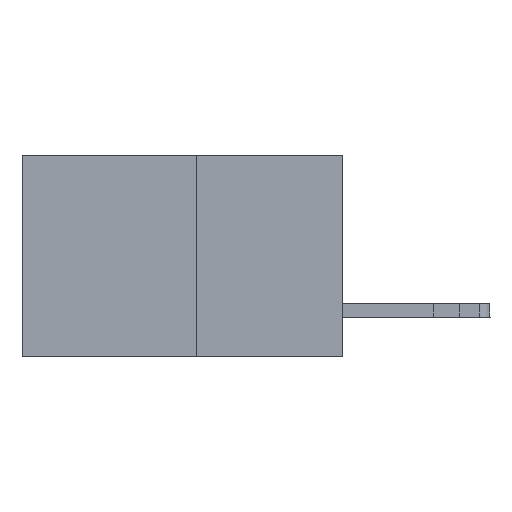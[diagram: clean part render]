
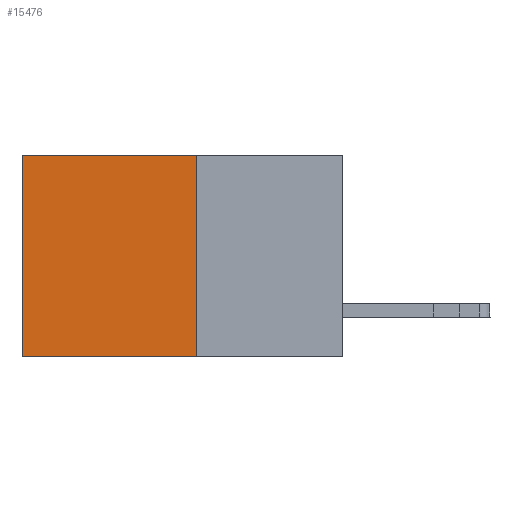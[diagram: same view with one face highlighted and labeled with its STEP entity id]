
A CAD part, left-side view. The second image highlights one B-rep face of the part: STEP entity #15476.
In plain terms, the highlighted planar face has unit normal (-1, 0, 0).
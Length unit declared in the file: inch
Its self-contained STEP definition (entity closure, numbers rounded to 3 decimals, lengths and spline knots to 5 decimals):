
#254 = EDGE_CURVE ( 'NONE', #26780, #20429, #19326, .T. ) ;
#1365 = VERTEX_POINT ( 'NONE', #3484 ) ;
#2814 = LINE ( 'NONE', #14311, #10953 ) ;
#2864 = EDGE_LOOP ( 'NONE', ( #21730, #12178, #21146, #21820 ) ) ;
#3484 = CARTESIAN_POINT ( 'NONE',  ( 0.277, 0.59, 0. ) ) ;
#6136 = VERTEX_POINT ( 'NONE', #21966 ) ;
#7174 = CARTESIAN_POINT ( 'NONE',  ( 0.277, 0.27, -0.37 ) ) ;
#8722 = CARTESIAN_POINT ( 'NONE',  ( 0.277, 0.27, -0.37 ) ) ;
#8841 = EDGE_CURVE ( 'NONE', #1365, #6136, #2814, .T. ) ;
#8931 = EDGE_CURVE ( 'NONE', #20429, #6136, #26790, .T. ) ;
#9670 = DIRECTION ( 'NONE',  ( 0., 1., 0. ) ) ;
#9918 = DIRECTION ( 'NONE',  ( 0., 1., 0. ) ) ;
#10953 = VECTOR ( 'NONE', #31587, 39.37008 ) ;
#11965 = EDGE_CURVE ( 'NONE', #26780, #1365, #26140, .T. ) ;
#12178 = ORIENTED_EDGE ( 'NONE', *, *, #8931, .F. ) ;
#12986 = VECTOR ( 'NONE', #9918, 39.37008 ) ;
#14311 = CARTESIAN_POINT ( 'NONE',  ( 0.277, 0.59, -0.37 ) ) ;
#14788 = CARTESIAN_POINT ( 'NONE',  ( 0.277, 0.27, 0. ) ) ;
#15362 = AXIS2_PLACEMENT_3D ( 'NONE', #22128, #19560, #27088 ) ;
#15476 = ADVANCED_FACE ( 'NONE', ( #15917 ), #24604, .F. ) ;
#15917 = FACE_OUTER_BOUND ( 'NONE', #2864, .T. ) ;
#19326 = LINE ( 'NONE', #31939, #30878 ) ;
#19484 = VECTOR ( 'NONE', #9670, 39.37008 ) ;
#19560 = DIRECTION ( 'NONE',  ( 1., 0., 0. ) ) ;
#20232 = CARTESIAN_POINT ( 'NONE',  ( 0.277, 0.27, 0. ) ) ;
#20429 = VERTEX_POINT ( 'NONE', #8722 ) ;
#21146 = ORIENTED_EDGE ( 'NONE', *, *, #254, .F. ) ;
#21730 = ORIENTED_EDGE ( 'NONE', *, *, #8841, .T. ) ;
#21820 = ORIENTED_EDGE ( 'NONE', *, *, #11965, .T. ) ;
#21966 = CARTESIAN_POINT ( 'NONE',  ( 0.277, 0.59, -0.37 ) ) ;
#22128 = CARTESIAN_POINT ( 'NONE',  ( 0.277, 0.27, -0.37 ) ) ;
#24604 = PLANE ( 'NONE',  #15362 ) ;
#26140 = LINE ( 'NONE', #14788, #12986 ) ;
#26780 = VERTEX_POINT ( 'NONE', #20232 ) ;
#26790 = LINE ( 'NONE', #7174, #19484 ) ;
#27088 = DIRECTION ( 'NONE',  ( 0., 0., -1. ) ) ;
#30878 = VECTOR ( 'NONE', #31700, 39.37008 ) ;
#31587 = DIRECTION ( 'NONE',  ( 0., 0., -1. ) ) ;
#31700 = DIRECTION ( 'NONE',  ( 0., 0., -1. ) ) ;
#31939 = CARTESIAN_POINT ( 'NONE',  ( 0.277, 0.27, -0.37 ) ) ;
